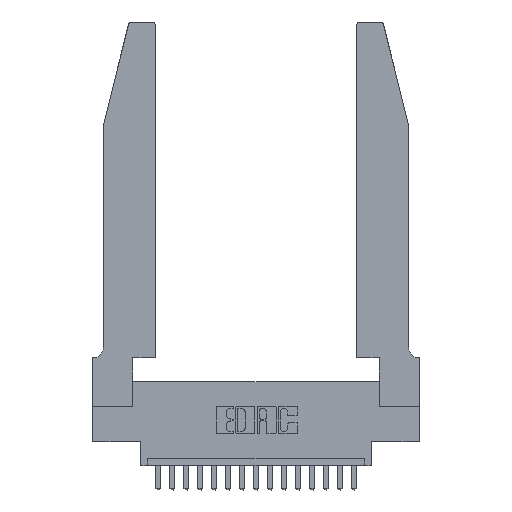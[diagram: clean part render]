
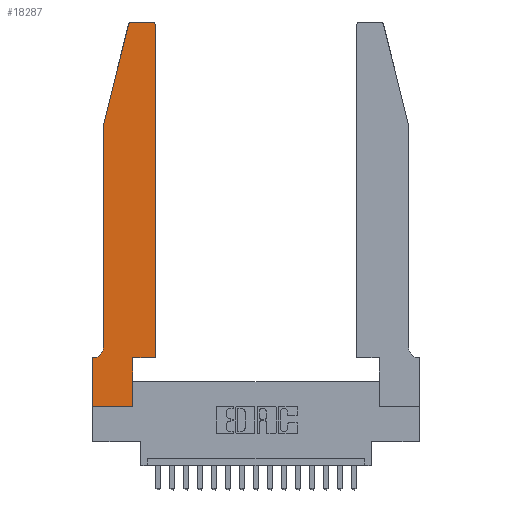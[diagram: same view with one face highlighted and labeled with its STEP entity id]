
A CAD part, top view. The second image highlights one B-rep face of the part: STEP entity #18287.
In plain terms, the highlighted planar face has unit normal (0, 0, 1).
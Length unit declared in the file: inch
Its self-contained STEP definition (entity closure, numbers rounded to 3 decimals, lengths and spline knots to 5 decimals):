
#180 = LINE ( 'NONE', #4834, #6006 ) ;
#374 = VECTOR ( 'NONE', #11579, 39.37008 ) ;
#688 = DIRECTION ( 'NONE',  ( 0., -1., 0. ) ) ;
#844 = EDGE_CURVE ( 'NONE', #9379, #2682, #9823, .T. ) ;
#1149 = ORIENTED_EDGE ( 'NONE', *, *, #9807, .T. ) ;
#1244 = ORIENTED_EDGE ( 'NONE', *, *, #7103, .T. ) ;
#1281 = VERTEX_POINT ( 'NONE', #7470 ) ;
#1372 = LINE ( 'NONE', #5612, #12261 ) ;
#1407 = LINE ( 'NONE', #2805, #3884 ) ;
#1623 = VERTEX_POINT ( 'NONE', #5635 ) ;
#1839 = VECTOR ( 'NONE', #15751, 39.37008 ) ;
#1894 = CARTESIAN_POINT ( 'NONE',  ( 0., 0., 0.37 ) ) ;
#2058 = VECTOR ( 'NONE', #688, 39.37008 ) ;
#2122 = CARTESIAN_POINT ( 'NONE',  ( 0.0755, 2., 0.37 ) ) ;
#2584 = ORIENTED_EDGE ( 'NONE', *, *, #4174, .T. ) ;
#2596 = EDGE_CURVE ( 'NONE', #18136, #9379, #14991, .T. ) ;
#2597 = CARTESIAN_POINT ( 'NONE',  ( 0.284, 2.75, 0.37 ) ) ;
#2661 = DIRECTION ( 'NONE',  ( 0., 1., 0. ) ) ;
#2666 = DIRECTION ( 'NONE',  ( 1., 0., 0. ) ) ;
#2682 = VERTEX_POINT ( 'NONE', #11997 ) ;
#2805 = CARTESIAN_POINT ( 'NONE',  ( 0.0755, 2., 0.37 ) ) ;
#2868 = PLANE ( 'NONE',  #17990 ) ;
#2963 = AXIS2_PLACEMENT_3D ( 'NONE', #18202, #11980, #10531 ) ;
#2998 = DIRECTION ( 'NONE',  ( 0., 0., 1. ) ) ;
#3033 = LINE ( 'NONE', #2122, #2058 ) ;
#3826 = EDGE_CURVE ( 'NONE', #1623, #18136, #7370, .T. ) ;
#3839 = EDGE_LOOP ( 'NONE', ( #19034, #16088, #10186, #1149, #2584, #15731, #18733, #18849, #1244, #10475, #4374, #14141 ) ) ;
#3884 = VECTOR ( 'NONE', #16815, 39.37008 ) ;
#3938 = DIRECTION ( 'NONE',  ( -1., 0., 0. ) ) ;
#4174 = EDGE_CURVE ( 'NONE', #13341, #13426, #5677, .T. ) ;
#4374 = ORIENTED_EDGE ( 'NONE', *, *, #6297, .T. ) ;
#4834 = CARTESIAN_POINT ( 'NONE',  ( 0.0755, 0.35, 0.37 ) ) ;
#5319 = LINE ( 'NONE', #18060, #18022 ) ;
#5578 = AXIS2_PLACEMENT_3D ( 'NONE', #6415, #12384, #15488 ) ;
#5612 = CARTESIAN_POINT ( 'NONE',  ( 0.4505, 0.35, 0.37 ) ) ;
#5635 = CARTESIAN_POINT ( 'NONE',  ( 0.4505, 2.72, 0.37 ) ) ;
#5677 = CIRCLE ( 'NONE', #2963, 0.07 ) ;
#5737 = DIRECTION ( 'NONE',  ( 0., 0., 1. ) ) ;
#6006 = VECTOR ( 'NONE', #6453, 39.37008 ) ;
#6207 = LINE ( 'NONE', #8570, #374 ) ;
#6297 = EDGE_CURVE ( 'NONE', #12322, #1623, #9674, .T. ) ;
#6311 = CARTESIAN_POINT ( 'NONE',  ( 0., 0., 0.37 ) ) ;
#6415 = CARTESIAN_POINT ( 'NONE',  ( 0.4205, 2.72, 0.37 ) ) ;
#6453 = DIRECTION ( 'NONE',  ( -1., 0., 0. ) ) ;
#7103 = EDGE_CURVE ( 'NONE', #1281, #15593, #5319, .T. ) ;
#7370 = CIRCLE ( 'NONE', #5578, 0.03 ) ;
#7470 = CARTESIAN_POINT ( 'NONE',  ( 0.2865, 0., 0.37 ) ) ;
#7702 = DIRECTION ( 'NONE',  ( 1., 0., 0. ) ) ;
#7756 = VERTEX_POINT ( 'NONE', #8396 ) ;
#7859 = EDGE_CURVE ( 'NONE', #13426, #7756, #180, .T. ) ;
#8124 = EDGE_CURVE ( 'NONE', #7756, #8756, #10338, .T. ) ;
#8396 = CARTESIAN_POINT ( 'NONE',  ( 0., 0.35, 0.37 ) ) ;
#8570 = CARTESIAN_POINT ( 'NONE',  ( 0., 0., 0.37 ) ) ;
#8756 = VERTEX_POINT ( 'NONE', #6311 ) ;
#9275 = CARTESIAN_POINT ( 'NONE',  ( 0.4205, 2.75, 0.37 ) ) ;
#9379 = VERTEX_POINT ( 'NONE', #2597 ) ;
#9674 = LINE ( 'NONE', #18228, #13267 ) ;
#9776 = EDGE_CURVE ( 'NONE', #8756, #1281, #6207, .T. ) ;
#9807 = EDGE_CURVE ( 'NONE', #10022, #13341, #3033, .T. ) ;
#9823 = CIRCLE ( 'NONE', #19279, 0.03 ) ;
#10022 = VERTEX_POINT ( 'NONE', #19591 ) ;
#10186 = ORIENTED_EDGE ( 'NONE', *, *, #12904, .T. ) ;
#10267 = CARTESIAN_POINT ( 'NONE',  ( 0.0055, 0.35, 0.37 ) ) ;
#10301 = CARTESIAN_POINT ( 'NONE',  ( 0.4505, 0.35, 0.37 ) ) ;
#10338 = LINE ( 'NONE', #1894, #1839 ) ;
#10475 = ORIENTED_EDGE ( 'NONE', *, *, #14020, .T. ) ;
#10531 = DIRECTION ( 'NONE',  ( -1., 0., 0. ) ) ;
#11579 = DIRECTION ( 'NONE',  ( 1., 0., 0. ) ) ;
#11935 = DIRECTION ( 'NONE',  ( 0., 1., 0. ) ) ;
#11980 = DIRECTION ( 'NONE',  ( 0., 0., -1. ) ) ;
#11997 = CARTESIAN_POINT ( 'NONE',  ( 0.25487, 2.72718, 0.37 ) ) ;
#12261 = VECTOR ( 'NONE', #13065, 39.37008 ) ;
#12322 = VERTEX_POINT ( 'NONE', #10301 ) ;
#12384 = DIRECTION ( 'NONE',  ( 0., 0., 1. ) ) ;
#12904 = EDGE_CURVE ( 'NONE', #2682, #10022, #1407, .T. ) ;
#13065 = DIRECTION ( 'NONE',  ( 1., 0., 0. ) ) ;
#13267 = VECTOR ( 'NONE', #11935, 39.37008 ) ;
#13312 = VECTOR ( 'NONE', #3938, 39.37008 ) ;
#13341 = VERTEX_POINT ( 'NONE', #17306 ) ;
#13426 = VERTEX_POINT ( 'NONE', #10267 ) ;
#13580 = CARTESIAN_POINT ( 'NONE',  ( 0., 0.35, 0.37 ) ) ;
#14020 = EDGE_CURVE ( 'NONE', #15593, #12322, #1372, .T. ) ;
#14141 = ORIENTED_EDGE ( 'NONE', *, *, #3826, .T. ) ;
#14357 = CARTESIAN_POINT ( 'NONE',  ( 0.2865, 0.35, 0.37 ) ) ;
#14991 = LINE ( 'NONE', #16153, #13312 ) ;
#15122 = CARTESIAN_POINT ( 'NONE',  ( 0.284, 2.72, 0.37 ) ) ;
#15488 = DIRECTION ( 'NONE',  ( 1., 0., 0. ) ) ;
#15593 = VERTEX_POINT ( 'NONE', #14357 ) ;
#15731 = ORIENTED_EDGE ( 'NONE', *, *, #7859, .T. ) ;
#15751 = DIRECTION ( 'NONE',  ( 0., -1., 0. ) ) ;
#16088 = ORIENTED_EDGE ( 'NONE', *, *, #844, .T. ) ;
#16153 = CARTESIAN_POINT ( 'NONE',  ( 0.2605, 2.75, 0.37 ) ) ;
#16815 = DIRECTION ( 'NONE',  ( -0.239, -0.971, 0. ) ) ;
#17306 = CARTESIAN_POINT ( 'NONE',  ( 0.0755, 0.42, 0.37 ) ) ;
#17398 = FACE_OUTER_BOUND ( 'NONE', #3839, .T. ) ;
#17990 = AXIS2_PLACEMENT_3D ( 'NONE', #13580, #5737, #2666 ) ;
#18022 = VECTOR ( 'NONE', #2661, 39.37008 ) ;
#18060 = CARTESIAN_POINT ( 'NONE',  ( 0.2865, 0.35, 0.37 ) ) ;
#18136 = VERTEX_POINT ( 'NONE', #9275 ) ;
#18202 = CARTESIAN_POINT ( 'NONE',  ( 0.0055, 0.42, 0.37 ) ) ;
#18228 = CARTESIAN_POINT ( 'NONE',  ( 0.4505, 0.35, 0.37 ) ) ;
#18287 = ADVANCED_FACE ( 'NONE', ( #17398 ), #2868, .T. ) ;
#18733 = ORIENTED_EDGE ( 'NONE', *, *, #8124, .T. ) ;
#18849 = ORIENTED_EDGE ( 'NONE', *, *, #9776, .T. ) ;
#19034 = ORIENTED_EDGE ( 'NONE', *, *, #2596, .T. ) ;
#19279 = AXIS2_PLACEMENT_3D ( 'NONE', #15122, #2998, #7702 ) ;
#19591 = CARTESIAN_POINT ( 'NONE',  ( 0.0755, 2., 0.37 ) ) ;
